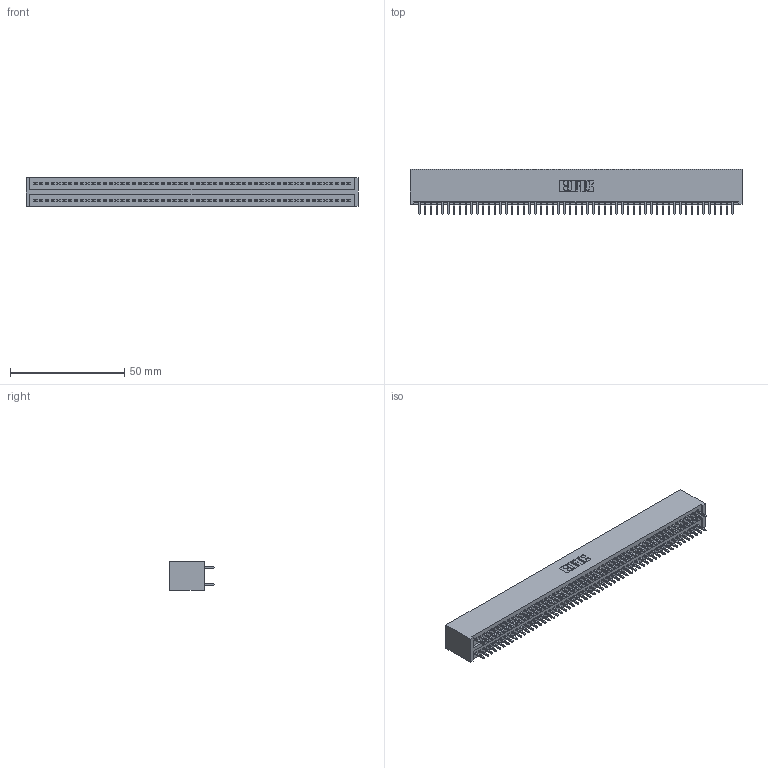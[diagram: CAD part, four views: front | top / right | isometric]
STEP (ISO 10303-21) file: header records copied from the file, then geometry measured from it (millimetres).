
FILE_DESCRIPTION (( 'STEP AP203' ), '1' );
FILE_NAME ('325-110-520-201.STEP', '2020-02-25T07:38:21', ( '' ), ( '' ), 'SwSTEP 2.0', 'SolidWorks 2016', '' );
FILE_SCHEMA (( 'CONFIG_CONTROL_DESIGN' ));
Length unit declared in the file: inch
Products named in the file (3): 325-110-520-201; 325 Part_Lugless; 325-292-001_325-293-120
Assembly tree (111 placements, depth 2):
  325-110-520-201
    325 Part_Lugless
    325-292-001_325-293-120  x110
Bounding box: 145.34 x 19.68 x 12.45 mm (x, y, z)
Volume: 19468.9 mm3; surface area: 24311.6 mm2
Topology: 111 solids, 111 shells, 5826 faces, 17337 edges, 11410 vertices
Faces by surface type: plane 4026, cylinder 1800
Entity records: 33443 total; most frequent: CARTESIAN_POINT 5526, ORIENTED_EDGE 5462, DIRECTION 4691, EDGE_CURVE 2731, VECTOR 2611, LINE 2611, VERTEX_POINT 1818, AXIS2_PLACEMENT_3D 1040
